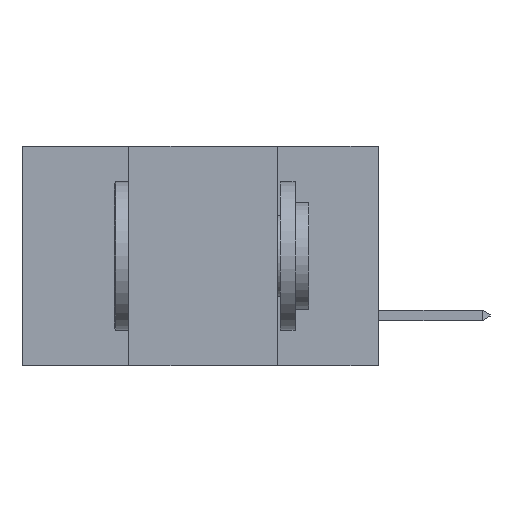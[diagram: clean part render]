
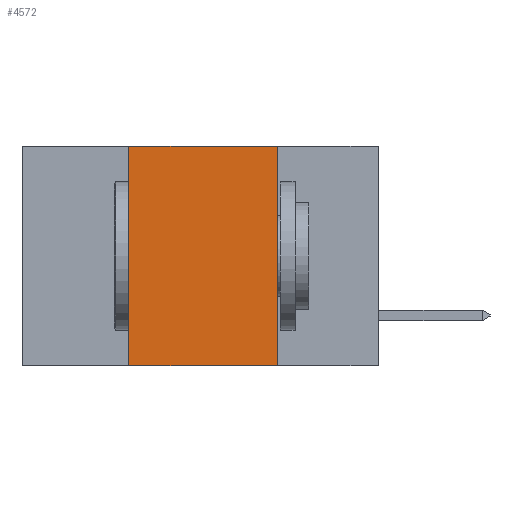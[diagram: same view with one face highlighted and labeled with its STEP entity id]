
A CAD part, left-side view. The second image highlights one B-rep face of the part: STEP entity #4572.
In plain terms, the highlighted planar face has unit normal (-1, 0, 0).
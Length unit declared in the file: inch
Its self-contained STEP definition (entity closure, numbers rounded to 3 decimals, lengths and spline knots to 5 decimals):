
#49 = CARTESIAN_POINT ( 'NONE',  ( 0., 0.6, 0. ) ) ;
#211 = PLANE ( 'NONE',  #11807 ) ;
#741 = VERTEX_POINT ( 'NONE', #12765 ) ;
#865 = CARTESIAN_POINT ( 'NONE',  ( 0., 0.42, 0. ) ) ;
#1203 = DIRECTION ( 'NONE',  ( 0., 0., -1. ) ) ;
#1691 = EDGE_CURVE ( 'NONE', #5651, #741, #12418, .T. ) ;
#1970 = EDGE_CURVE ( 'NONE', #741, #7609, #14119, .T. ) ;
#1989 = EDGE_CURVE ( 'NONE', #9393, #5651, #11750, .T. ) ;
#1993 = EDGE_CURVE ( 'NONE', #9393, #7609, #11105, .T. ) ;
#2726 = ORIENTED_EDGE ( 'NONE', *, *, #1691, .F. ) ;
#2731 = VECTOR ( 'NONE', #8830, 39.37008 ) ;
#3816 = VECTOR ( 'NONE', #9666, 39.37008 ) ;
#4572 = ADVANCED_FACE ( 'NONE', ( #8326 ), #211, .F. ) ;
#5651 = VERTEX_POINT ( 'NONE', #7373 ) ;
#5831 = ORIENTED_EDGE ( 'NONE', *, *, #1993, .T. ) ;
#6022 = CARTESIAN_POINT ( 'NONE',  ( 0., 0.17, -0.37 ) ) ;
#6122 = EDGE_LOOP ( 'NONE', ( #7071, #2726, #7027, #5831 ) ) ;
#7027 = ORIENTED_EDGE ( 'NONE', *, *, #1989, .F. ) ;
#7062 = CARTESIAN_POINT ( 'NONE',  ( 0., 0.6, -0.37 ) ) ;
#7071 = ORIENTED_EDGE ( 'NONE', *, *, #1970, .F. ) ;
#7373 = CARTESIAN_POINT ( 'NONE',  ( 0., 0.42, 0. ) ) ;
#7609 = VERTEX_POINT ( 'NONE', #6022 ) ;
#8326 = FACE_OUTER_BOUND ( 'NONE', #6122, .T. ) ;
#8796 = DIRECTION ( 'NONE',  ( 0., -1., 0. ) ) ;
#8830 = DIRECTION ( 'NONE',  ( 0., 0., 1. ) ) ;
#9393 = VERTEX_POINT ( 'NONE', #13854 ) ;
#9661 = CARTESIAN_POINT ( 'NONE',  ( 0., 0.6, 0. ) ) ;
#9666 = DIRECTION ( 'NONE',  ( 0., -1., 0. ) ) ;
#10791 = VECTOR ( 'NONE', #8796, 39.37008 ) ;
#11105 = LINE ( 'NONE', #7062, #10791 ) ;
#11732 = DIRECTION ( 'NONE',  ( 0., 0., -1. ) ) ;
#11750 = LINE ( 'NONE', #865, #2731 ) ;
#11807 = AXIS2_PLACEMENT_3D ( 'NONE', #49, #12523, #11732 ) ;
#12418 = LINE ( 'NONE', #9661, #3816 ) ;
#12523 = DIRECTION ( 'NONE',  ( 1., 0., 0. ) ) ;
#12765 = CARTESIAN_POINT ( 'NONE',  ( 0., 0.17, 0. ) ) ;
#13177 = CARTESIAN_POINT ( 'NONE',  ( 0., 0.17, 0. ) ) ;
#13815 = VECTOR ( 'NONE', #1203, 39.37008 ) ;
#13854 = CARTESIAN_POINT ( 'NONE',  ( 0., 0.42, -0.37 ) ) ;
#14119 = LINE ( 'NONE', #13177, #13815 ) ;
